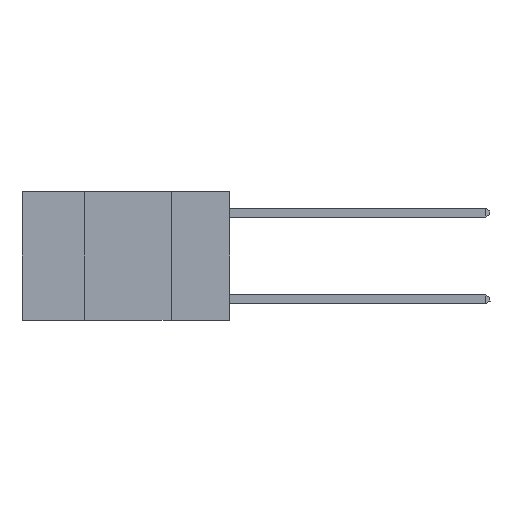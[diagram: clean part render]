
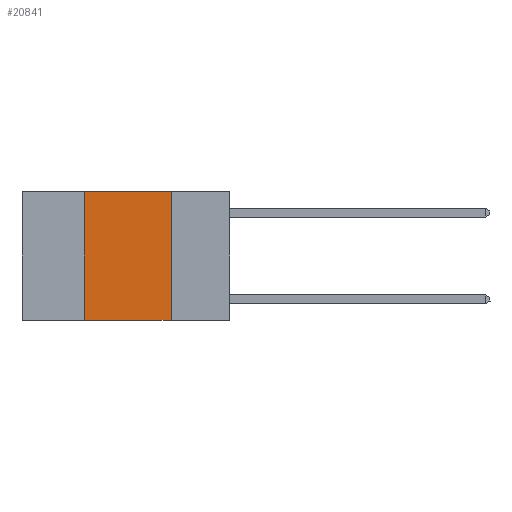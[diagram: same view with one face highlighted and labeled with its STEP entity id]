
A CAD part, left-side view. The second image highlights one B-rep face of the part: STEP entity #20841.
In plain terms, the highlighted planar face has unit normal (-1, 0, 0).
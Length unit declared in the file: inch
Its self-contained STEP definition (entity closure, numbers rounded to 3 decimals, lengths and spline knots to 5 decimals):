
#449 = PLANE ( 'NONE',  #15231 ) ;
#522 = DIRECTION ( 'NONE',  ( 0., 0., -1. ) ) ;
#1685 = DIRECTION ( 'NONE',  ( 0., 0., 1. ) ) ;
#1859 = CARTESIAN_POINT ( 'NONE',  ( 0., 0.6, 0. ) ) ;
#3285 = VERTEX_POINT ( 'NONE', #11052 ) ;
#3703 = ORIENTED_EDGE ( 'NONE', *, *, #24009, .F. ) ;
#4465 = LINE ( 'NONE', #23961, #13736 ) ;
#5156 = EDGE_LOOP ( 'NONE', ( #22289, #3703, #8613, #13534 ) ) ;
#5515 = DIRECTION ( 'NONE',  ( 0., -1., 0. ) ) ;
#5623 = VERTEX_POINT ( 'NONE', #10079 ) ;
#5640 = DIRECTION ( 'NONE',  ( 0., -1., 0. ) ) ;
#5952 = EDGE_CURVE ( 'NONE', #5623, #3285, #12072, .T. ) ;
#7210 = EDGE_CURVE ( 'NONE', #5623, #17779, #4465, .T. ) ;
#7336 = LINE ( 'NONE', #19792, #21548 ) ;
#8052 = FACE_OUTER_BOUND ( 'NONE', #5156, .T. ) ;
#8415 = EDGE_CURVE ( 'NONE', #15262, #3285, #7336, .T. ) ;
#8613 = ORIENTED_EDGE ( 'NONE', *, *, #7210, .F. ) ;
#10079 = CARTESIAN_POINT ( 'NONE',  ( 0., 0.42, -0.37 ) ) ;
#10516 = DIRECTION ( 'NONE',  ( 0., 0., -1. ) ) ;
#11052 = CARTESIAN_POINT ( 'NONE',  ( 0., 0.17, -0.37 ) ) ;
#11686 = DIRECTION ( 'NONE',  ( 1., 0., 0. ) ) ;
#12072 = LINE ( 'NONE', #14771, #16433 ) ;
#12490 = CARTESIAN_POINT ( 'NONE',  ( 0., 0.17, 0. ) ) ;
#13534 = ORIENTED_EDGE ( 'NONE', *, *, #5952, .T. ) ;
#13736 = VECTOR ( 'NONE', #1685, 39.37008 ) ;
#13976 = CARTESIAN_POINT ( 'NONE',  ( 0., 0.42, 0. ) ) ;
#14771 = CARTESIAN_POINT ( 'NONE',  ( 0., 0.6, -0.37 ) ) ;
#15231 = AXIS2_PLACEMENT_3D ( 'NONE', #20903, #11686, #522 ) ;
#15262 = VERTEX_POINT ( 'NONE', #12490 ) ;
#15862 = VECTOR ( 'NONE', #5640, 39.37008 ) ;
#16433 = VECTOR ( 'NONE', #5515, 39.37008 ) ;
#17779 = VERTEX_POINT ( 'NONE', #13976 ) ;
#19792 = CARTESIAN_POINT ( 'NONE',  ( 0., 0.17, 0. ) ) ;
#20841 = ADVANCED_FACE ( 'NONE', ( #8052 ), #449, .F. ) ;
#20860 = LINE ( 'NONE', #1859, #15862 ) ;
#20903 = CARTESIAN_POINT ( 'NONE',  ( 0., 0.6, 0. ) ) ;
#21548 = VECTOR ( 'NONE', #10516, 39.37008 ) ;
#22289 = ORIENTED_EDGE ( 'NONE', *, *, #8415, .F. ) ;
#23961 = CARTESIAN_POINT ( 'NONE',  ( 0., 0.42, 0. ) ) ;
#24009 = EDGE_CURVE ( 'NONE', #17779, #15262, #20860, .T. ) ;
